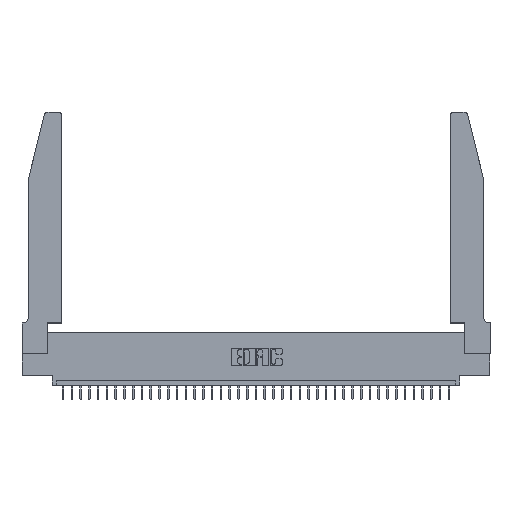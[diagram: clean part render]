
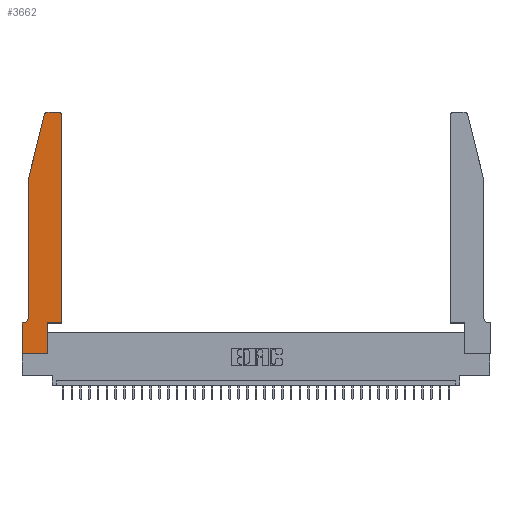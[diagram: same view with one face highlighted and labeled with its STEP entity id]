
A CAD part, top view. The second image highlights one B-rep face of the part: STEP entity #3662.
In plain terms, the highlighted planar face has unit normal (0, 0, 1).
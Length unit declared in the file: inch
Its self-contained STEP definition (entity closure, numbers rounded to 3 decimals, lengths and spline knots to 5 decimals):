
#73 = VECTOR ( 'NONE', #23114, 39.37008 ) ;
#1162 = EDGE_CURVE ( 'NONE', #11676, #17465, #37653, .T. ) ;
#1297 = CARTESIAN_POINT ( 'NONE',  ( 0.0755, 2., 0.37 ) ) ;
#2867 = CARTESIAN_POINT ( 'NONE',  ( 0.4205, 2.72, 0.37 ) ) ;
#3141 = EDGE_CURVE ( 'NONE', #31137, #34198, #23829, .T. ) ;
#3311 = EDGE_CURVE ( 'NONE', #4754, #19791, #25252, .T. ) ;
#3662 = ADVANCED_FACE ( 'NONE', ( #29367 ), #32466, .T. ) ;
#3699 = LINE ( 'NONE', #25664, #22357 ) ;
#3805 = CARTESIAN_POINT ( 'NONE',  ( 0.2605, 2.75, 0.37 ) ) ;
#4119 = CARTESIAN_POINT ( 'NONE',  ( 0.25487, 2.72718, 0.37 ) ) ;
#4754 = VERTEX_POINT ( 'NONE', #31542 ) ;
#5285 = DIRECTION ( 'NONE',  ( 1., 0., 0. ) ) ;
#5593 = ORIENTED_EDGE ( 'NONE', *, *, #16365, .T. ) ;
#5810 = EDGE_CURVE ( 'NONE', #34198, #12964, #37596, .T. ) ;
#5843 = CARTESIAN_POINT ( 'NONE',  ( 0., 0., 0.37 ) ) ;
#5905 = EDGE_CURVE ( 'NONE', #32438, #4754, #21790, .T. ) ;
#5974 = ORIENTED_EDGE ( 'NONE', *, *, #5810, .T. ) ;
#6916 = DIRECTION ( 'NONE',  ( 0., 0., 1. ) ) ;
#6979 = CARTESIAN_POINT ( 'NONE',  ( 0.284, 2.75, 0.37 ) ) ;
#8281 = ORIENTED_EDGE ( 'NONE', *, *, #25891, .T. ) ;
#8857 = EDGE_CURVE ( 'NONE', #8979, #9006, #3699, .T. ) ;
#8979 = VERTEX_POINT ( 'NONE', #36972 ) ;
#9006 = VERTEX_POINT ( 'NONE', #31417 ) ;
#9066 = ORIENTED_EDGE ( 'NONE', *, *, #5905, .T. ) ;
#9346 = ORIENTED_EDGE ( 'NONE', *, *, #1162, .T. ) ;
#10271 = CARTESIAN_POINT ( 'NONE',  ( 0.4505, 0.35, 0.37 ) ) ;
#10438 = DIRECTION ( 'NONE',  ( 1., 0., 0. ) ) ;
#11041 = CARTESIAN_POINT ( 'NONE',  ( 0.0055, 0.35, 0.37 ) ) ;
#11357 = DIRECTION ( 'NONE',  ( 0., 0., 1. ) ) ;
#11614 = DIRECTION ( 'NONE',  ( 1., 0., 0. ) ) ;
#11676 = VERTEX_POINT ( 'NONE', #4119 ) ;
#11845 = DIRECTION ( 'NONE',  ( 0., 0., -1. ) ) ;
#12408 = AXIS2_PLACEMENT_3D ( 'NONE', #2867, #11357, #10438 ) ;
#12865 = DIRECTION ( 'NONE',  ( 0., -1., 0. ) ) ;
#12964 = VERTEX_POINT ( 'NONE', #14695 ) ;
#13534 = ORIENTED_EDGE ( 'NONE', *, *, #36912, .T. ) ;
#13981 = DIRECTION ( 'NONE',  ( -0.239, -0.971, 0. ) ) ;
#14051 = EDGE_CURVE ( 'NONE', #19791, #16536, #36285, .T. ) ;
#14695 = CARTESIAN_POINT ( 'NONE',  ( 0., 0.35, 0.37 ) ) ;
#14875 = VECTOR ( 'NONE', #32634, 39.37008 ) ;
#15314 = VECTOR ( 'NONE', #37411, 39.37008 ) ;
#15563 = CARTESIAN_POINT ( 'NONE',  ( 0.4205, 2.75, 0.37 ) ) ;
#16365 = EDGE_CURVE ( 'NONE', #17465, #31137, #23777, .T. ) ;
#16375 = DIRECTION ( 'NONE',  ( 1., 0., 0. ) ) ;
#16536 = VERTEX_POINT ( 'NONE', #6979 ) ;
#16609 = ORIENTED_EDGE ( 'NONE', *, *, #14051, .T. ) ;
#17145 = LINE ( 'NONE', #27377, #35154 ) ;
#17171 = AXIS2_PLACEMENT_3D ( 'NONE', #20674, #11845, #26246 ) ;
#17465 = VERTEX_POINT ( 'NONE', #1297 ) ;
#17468 = DIRECTION ( 'NONE',  ( 0., 0., 1. ) ) ;
#17527 = CARTESIAN_POINT ( 'NONE',  ( 0.0755, 2., 0.37 ) ) ;
#18648 = DIRECTION ( 'NONE',  ( -1., 0., 0. ) ) ;
#18712 = VECTOR ( 'NONE', #18648, 39.37008 ) ;
#19325 = CARTESIAN_POINT ( 'NONE',  ( 0.4505, 0.35, 0.37 ) ) ;
#19791 = VERTEX_POINT ( 'NONE', #15563 ) ;
#20135 = CARTESIAN_POINT ( 'NONE',  ( 0.0755, 2., 0.37 ) ) ;
#20567 = EDGE_CURVE ( 'NONE', #12964, #8979, #26734, .T. ) ;
#20674 = CARTESIAN_POINT ( 'NONE',  ( 0.0055, 0.42, 0.37 ) ) ;
#21790 = LINE ( 'NONE', #19325, #14875 ) ;
#21797 = ORIENTED_EDGE ( 'NONE', *, *, #3311, .T. ) ;
#21804 = AXIS2_PLACEMENT_3D ( 'NONE', #24726, #6916, #33257 ) ;
#22357 = VECTOR ( 'NONE', #5285, 39.37008 ) ;
#23035 = DIRECTION ( 'NONE',  ( 0., 1., 0. ) ) ;
#23114 = DIRECTION ( 'NONE',  ( 0., -1., 0. ) ) ;
#23418 = CARTESIAN_POINT ( 'NONE',  ( 0.2865, 0.35, 0.37 ) ) ;
#23441 = ORIENTED_EDGE ( 'NONE', *, *, #8857, .T. ) ;
#23777 = LINE ( 'NONE', #20135, #73 ) ;
#23829 = CIRCLE ( 'NONE', #17171, 0.07 ) ;
#24163 = VECTOR ( 'NONE', #13981, 39.37008 ) ;
#24726 = CARTESIAN_POINT ( 'NONE',  ( 0.284, 2.72, 0.37 ) ) ;
#25252 = CIRCLE ( 'NONE', #12408, 0.03 ) ;
#25664 = CARTESIAN_POINT ( 'NONE',  ( 0., 0., 0.37 ) ) ;
#25696 = ORIENTED_EDGE ( 'NONE', *, *, #35310, .T. ) ;
#25891 = EDGE_CURVE ( 'NONE', #31734, #32438, #17145, .T. ) ;
#26246 = DIRECTION ( 'NONE',  ( -1., 0., 0. ) ) ;
#26734 = LINE ( 'NONE', #5843, #30893 ) ;
#27377 = CARTESIAN_POINT ( 'NONE',  ( 0.4505, 0.35, 0.37 ) ) ;
#28890 = CARTESIAN_POINT ( 'NONE',  ( 0.0755, 0.42, 0.37 ) ) ;
#29367 = FACE_OUTER_BOUND ( 'NONE', #30471, .T. ) ;
#29603 = CARTESIAN_POINT ( 'NONE',  ( 0., 0.35, 0.37 ) ) ;
#30471 = EDGE_LOOP ( 'NONE', ( #16609, #13534, #9346, #5593, #35344, #5974, #32010, #23441, #25696, #8281, #9066, #21797 ) ) ;
#30634 = CARTESIAN_POINT ( 'NONE',  ( 0.2865, 0.35, 0.37 ) ) ;
#30893 = VECTOR ( 'NONE', #12865, 39.37008 ) ;
#31137 = VERTEX_POINT ( 'NONE', #28890 ) ;
#31357 = CIRCLE ( 'NONE', #21804, 0.03 ) ;
#31417 = CARTESIAN_POINT ( 'NONE',  ( 0.2865, 0., 0.37 ) ) ;
#31488 = LINE ( 'NONE', #23418, #34706 ) ;
#31542 = CARTESIAN_POINT ( 'NONE',  ( 0.4505, 2.72, 0.37 ) ) ;
#31734 = VERTEX_POINT ( 'NONE', #30634 ) ;
#32010 = ORIENTED_EDGE ( 'NONE', *, *, #20567, .T. ) ;
#32297 = AXIS2_PLACEMENT_3D ( 'NONE', #29603, #17468, #11614 ) ;
#32438 = VERTEX_POINT ( 'NONE', #10271 ) ;
#32466 = PLANE ( 'NONE',  #32297 ) ;
#32634 = DIRECTION ( 'NONE',  ( 0., 1., 0. ) ) ;
#33257 = DIRECTION ( 'NONE',  ( 1., 0., 0. ) ) ;
#34198 = VERTEX_POINT ( 'NONE', #11041 ) ;
#34706 = VECTOR ( 'NONE', #23035, 39.37008 ) ;
#35154 = VECTOR ( 'NONE', #16375, 39.37008 ) ;
#35310 = EDGE_CURVE ( 'NONE', #9006, #31734, #31488, .T. ) ;
#35344 = ORIENTED_EDGE ( 'NONE', *, *, #3141, .T. ) ;
#36285 = LINE ( 'NONE', #3805, #18712 ) ;
#36346 = CARTESIAN_POINT ( 'NONE',  ( 0.0755, 0.35, 0.37 ) ) ;
#36912 = EDGE_CURVE ( 'NONE', #16536, #11676, #31357, .T. ) ;
#36972 = CARTESIAN_POINT ( 'NONE',  ( 0., 0., 0.37 ) ) ;
#37411 = DIRECTION ( 'NONE',  ( -1., 0., 0. ) ) ;
#37596 = LINE ( 'NONE', #36346, #15314 ) ;
#37653 = LINE ( 'NONE', #17527, #24163 ) ;
